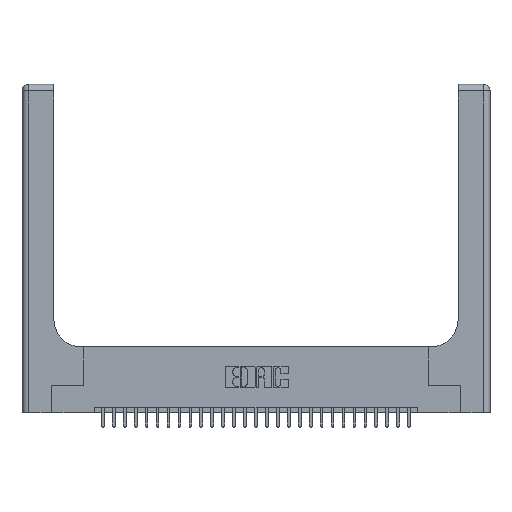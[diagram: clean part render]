
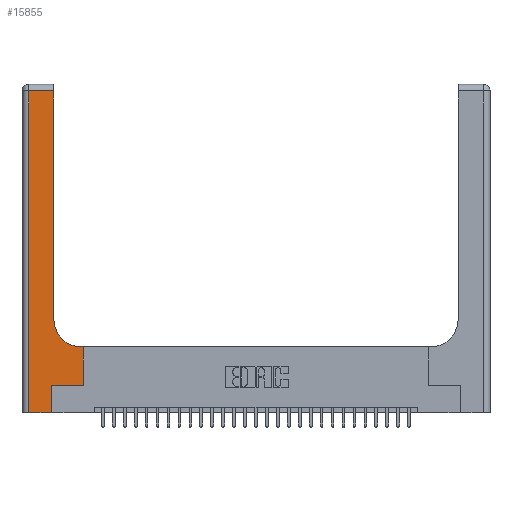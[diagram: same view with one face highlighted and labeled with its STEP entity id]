
A CAD part, top view. The second image highlights one B-rep face of the part: STEP entity #15855.
In plain terms, the highlighted planar face has unit normal (0, 0, 1).
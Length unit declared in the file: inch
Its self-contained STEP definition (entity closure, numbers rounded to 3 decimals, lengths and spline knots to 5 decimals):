
#224 = DIRECTION ( 'NONE',  ( 0., 0., -1. ) ) ;
#342 = DIRECTION ( 'NONE',  ( 1., 0., 0. ) ) ;
#446 = DIRECTION ( 'NONE',  ( 1., 0., 0. ) ) ;
#497 = EDGE_CURVE ( 'NONE', #1150, #6740, #3431, .T. ) ;
#599 = DIRECTION ( 'NONE',  ( -1., 0., 0. ) ) ;
#625 = DIRECTION ( 'NONE',  ( -1., 0., 0. ) ) ;
#1150 = VERTEX_POINT ( 'NONE', #11646 ) ;
#3348 = VECTOR ( 'NONE', #25661, 39.37008 ) ;
#3431 = LINE ( 'NONE', #7304, #23529 ) ;
#4846 = LINE ( 'NONE', #28907, #24956 ) ;
#5537 = ORIENTED_EDGE ( 'NONE', *, *, #21538, .T. ) ;
#5899 = CARTESIAN_POINT ( 'NONE',  ( 0.269, 0.25, 0.37 ) ) ;
#6442 = ORIENTED_EDGE ( 'NONE', *, *, #15323, .T. ) ;
#6740 = VERTEX_POINT ( 'NONE', #8754 ) ;
#6811 = VECTOR ( 'NONE', #21966, 39.37008 ) ;
#7207 = FACE_OUTER_BOUND ( 'NONE', #9995, .T. ) ;
#7304 = CARTESIAN_POINT ( 'NONE',  ( 0., 2.94, 0.37 ) ) ;
#7373 = AXIS2_PLACEMENT_3D ( 'NONE', #18836, #16252, #342 ) ;
#7418 = ORIENTED_EDGE ( 'NONE', *, *, #8657, .T. ) ;
#7791 = CARTESIAN_POINT ( 'NONE',  ( 0.5585, 0.25, 0.37 ) ) ;
#8606 = CARTESIAN_POINT ( 'NONE',  ( 0.269, 0.25, 0.37 ) ) ;
#8657 = EDGE_CURVE ( 'NONE', #25193, #29624, #11794, .T. ) ;
#8754 = CARTESIAN_POINT ( 'NONE',  ( 0.06, 2.94, 0.37 ) ) ;
#8844 = EDGE_CURVE ( 'NONE', #12492, #17062, #23967, .T. ) ;
#9345 = PLANE ( 'NONE',  #21357 ) ;
#9995 = EDGE_LOOP ( 'NONE', ( #13681, #14781, #6442, #5537, #18837, #16778, #7418, #22170, #15671 ) ) ;
#10111 = CARTESIAN_POINT ( 'NONE',  ( 0.2915, 0.85, 0.37 ) ) ;
#10162 = LINE ( 'NONE', #25562, #3348 ) ;
#10580 = CARTESIAN_POINT ( 'NONE',  ( 0.269, 0., 0.37 ) ) ;
#10812 = CARTESIAN_POINT ( 'NONE',  ( 0.5585, 0.25, 0.37 ) ) ;
#11646 = CARTESIAN_POINT ( 'NONE',  ( 0.2915, 2.94, 0.37 ) ) ;
#11794 = LINE ( 'NONE', #10812, #26513 ) ;
#12492 = VERTEX_POINT ( 'NONE', #19344 ) ;
#12578 = EDGE_CURVE ( 'NONE', #17062, #1150, #19838, .T. ) ;
#12795 = CARTESIAN_POINT ( 'NONE',  ( 0.5585, 0.6, 0.37 ) ) ;
#13132 = DIRECTION ( 'NONE',  ( 0., 1., 0. ) ) ;
#13681 = ORIENTED_EDGE ( 'NONE', *, *, #12578, .T. ) ;
#13832 = VERTEX_POINT ( 'NONE', #10580 ) ;
#14000 = CARTESIAN_POINT ( 'NONE',  ( 0., 3., 0.37 ) ) ;
#14474 = VECTOR ( 'NONE', #24738, 39.37008 ) ;
#14685 = VERTEX_POINT ( 'NONE', #23282 ) ;
#14781 = ORIENTED_EDGE ( 'NONE', *, *, #497, .T. ) ;
#15323 = EDGE_CURVE ( 'NONE', #6740, #14685, #10162, .T. ) ;
#15671 = ORIENTED_EDGE ( 'NONE', *, *, #8844, .T. ) ;
#15855 = ADVANCED_FACE ( 'NONE', ( #7207 ), #9345, .F. ) ;
#16155 = CARTESIAN_POINT ( 'NONE',  ( 0.2915, 0.6, 0.37 ) ) ;
#16252 = DIRECTION ( 'NONE',  ( 0., 0., -1. ) ) ;
#16636 = DIRECTION ( 'NONE',  ( -1., 0., 0. ) ) ;
#16778 = ORIENTED_EDGE ( 'NONE', *, *, #25300, .T. ) ;
#17062 = VERTEX_POINT ( 'NONE', #10111 ) ;
#17084 = LINE ( 'NONE', #27746, #27797 ) ;
#17852 = CARTESIAN_POINT ( 'NONE',  ( 0.2915, 3., 0.37 ) ) ;
#18203 = VECTOR ( 'NONE', #16636, 39.37008 ) ;
#18615 = VERTEX_POINT ( 'NONE', #8606 ) ;
#18836 = CARTESIAN_POINT ( 'NONE',  ( 0.5415, 0.85, 0.37 ) ) ;
#18837 = ORIENTED_EDGE ( 'NONE', *, *, #28529, .T. ) ;
#19067 = LINE ( 'NONE', #5899, #6811 ) ;
#19344 = CARTESIAN_POINT ( 'NONE',  ( 0.5415, 0.6, 0.37 ) ) ;
#19838 = LINE ( 'NONE', #17852, #14474 ) ;
#21357 = AXIS2_PLACEMENT_3D ( 'NONE', #14000, #224, #625 ) ;
#21538 = EDGE_CURVE ( 'NONE', #14685, #13832, #17084, .T. ) ;
#21966 = DIRECTION ( 'NONE',  ( 1., 0., 0. ) ) ;
#22170 = ORIENTED_EDGE ( 'NONE', *, *, #27097, .T. ) ;
#23282 = CARTESIAN_POINT ( 'NONE',  ( 0.06, 0., 0.37 ) ) ;
#23529 = VECTOR ( 'NONE', #599, 39.37008 ) ;
#23967 = CIRCLE ( 'NONE', #7373, 0.25 ) ;
#24738 = DIRECTION ( 'NONE',  ( 0., 1., 0. ) ) ;
#24956 = VECTOR ( 'NONE', #26233, 39.37008 ) ;
#25193 = VERTEX_POINT ( 'NONE', #7791 ) ;
#25300 = EDGE_CURVE ( 'NONE', #18615, #25193, #19067, .T. ) ;
#25562 = CARTESIAN_POINT ( 'NONE',  ( 0.06, 3., 0.37 ) ) ;
#25661 = DIRECTION ( 'NONE',  ( 0., -1., 0. ) ) ;
#26233 = DIRECTION ( 'NONE',  ( 0., 1., 0. ) ) ;
#26513 = VECTOR ( 'NONE', #13132, 39.37008 ) ;
#27097 = EDGE_CURVE ( 'NONE', #29624, #12492, #27151, .T. ) ;
#27151 = LINE ( 'NONE', #16155, #18203 ) ;
#27746 = CARTESIAN_POINT ( 'NONE',  ( 0., 0., 0.37 ) ) ;
#27797 = VECTOR ( 'NONE', #446, 39.37008 ) ;
#28529 = EDGE_CURVE ( 'NONE', #13832, #18615, #4846, .T. ) ;
#28907 = CARTESIAN_POINT ( 'NONE',  ( 0.269, 0., 0.37 ) ) ;
#29624 = VERTEX_POINT ( 'NONE', #12795 ) ;
